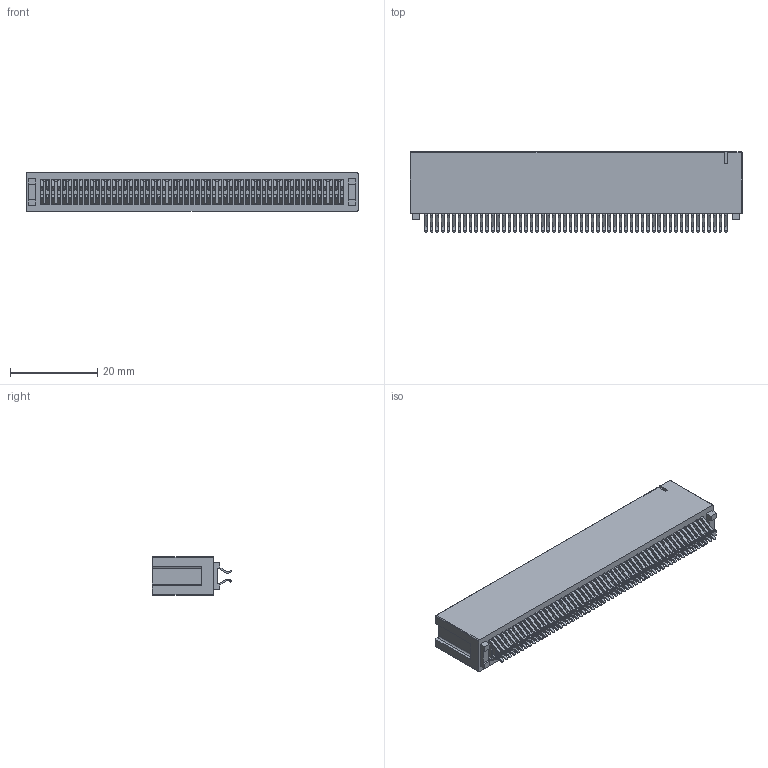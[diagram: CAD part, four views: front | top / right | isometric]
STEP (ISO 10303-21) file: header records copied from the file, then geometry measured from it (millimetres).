
FILE_DESCRIPTION (( 'STEP AP203' ), '1' );
FILE_NAME ('302-110-356-201.STEP', '2024-04-06T14:36:26', ( '' ), ( '' ), 'SwSTEP 2.0', 'SolidWorks 2023', '' );
FILE_SCHEMA (( 'CONFIG_CONTROL_DESIGN' ));
Length unit declared in the file: millimetre
Products named in the file (3): Contact_302-290-X56; HSG_Vertical HSG; 302-110-356-201
Assembly tree (111 placements, depth 2):
  302-110-356-201
    HSG_Vertical HSG
    Contact_302-290-X56  x110
Bounding box: 75.95 x 18.3 x 8.88 mm (x, y, z)
Volume: 5808 mm3; surface area: 16678.8 mm2
Topology: 111 solids, 111 shells, 5291 faces, 15788 edges, 10444 vertices
Faces by surface type: plane 3514, cylinder 1773, sphere 4
Entity records: 41445 total; most frequent: ORIENTED_EDGE 7152, CARTESIAN_POINT 7019, DIRECTION 5716, EDGE_CURVE 3576, VECTOR 3518, LINE 3518, VERTEX_POINT 2378, EDGE_LOOP 1100
